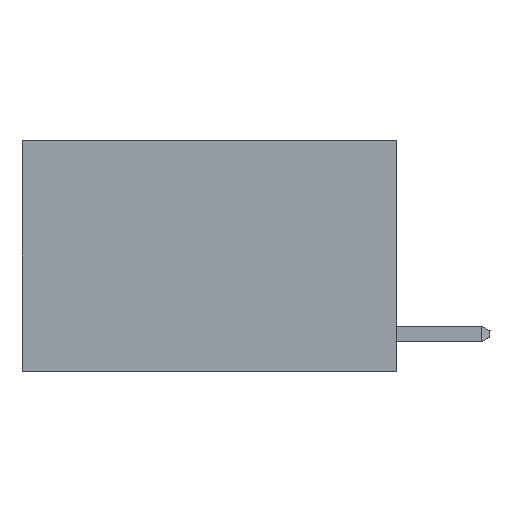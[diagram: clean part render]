
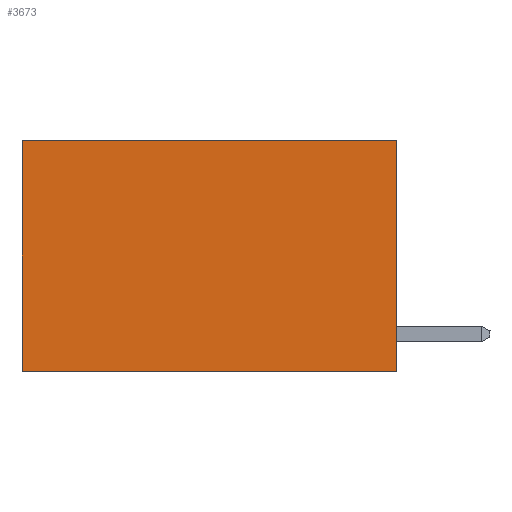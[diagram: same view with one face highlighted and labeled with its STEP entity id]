
A CAD part, left-side view. The second image highlights one B-rep face of the part: STEP entity #3673.
In plain terms, the highlighted planar face has unit normal (-1, 0, 0).
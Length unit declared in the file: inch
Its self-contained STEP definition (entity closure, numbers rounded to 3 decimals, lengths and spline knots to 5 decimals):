
#211 = LINE ( 'NONE', #10325, #7303 ) ;
#1098 = LINE ( 'NONE', #10090, #13282 ) ;
#1186 = PLANE ( 'NONE',  #10611 ) ;
#1551 = ORIENTED_EDGE ( 'NONE', *, *, #12879, .T. ) ;
#2731 = EDGE_LOOP ( 'NONE', ( #1551, #8288, #7806, #10249 ) ) ;
#3109 = VERTEX_POINT ( 'NONE', #12975 ) ;
#3256 = DIRECTION ( 'NONE',  ( 0., 0., -1. ) ) ;
#3499 = CARTESIAN_POINT ( 'NONE',  ( 0.2625, 0., 0. ) ) ;
#3673 = ADVANCED_FACE ( 'NONE', ( #4458 ), #1186, .F. ) ;
#4458 = FACE_OUTER_BOUND ( 'NONE', #2731, .T. ) ;
#4894 = DIRECTION ( 'NONE',  ( 0., 1., 0. ) ) ;
#4955 = VERTEX_POINT ( 'NONE', #10124 ) ;
#5085 = CARTESIAN_POINT ( 'NONE',  ( 0.2625, 0.6, -0.37 ) ) ;
#5705 = DIRECTION ( 'NONE',  ( 0., 0., -1. ) ) ;
#6504 = LINE ( 'NONE', #12105, #10419 ) ;
#6715 = CARTESIAN_POINT ( 'NONE',  ( 0.2625, 0., 0. ) ) ;
#6963 = DIRECTION ( 'NONE',  ( 1., 0., 0. ) ) ;
#7303 = VECTOR ( 'NONE', #4894, 39.37008 ) ;
#7806 = ORIENTED_EDGE ( 'NONE', *, *, #11820, .F. ) ;
#8288 = ORIENTED_EDGE ( 'NONE', *, *, #8401, .F. ) ;
#8401 = EDGE_CURVE ( 'NONE', #4955, #13321, #211, .T. ) ;
#9069 = LINE ( 'NONE', #6715, #12282 ) ;
#9902 = CARTESIAN_POINT ( 'NONE',  ( 0.2625, 0.6, 0. ) ) ;
#10090 = CARTESIAN_POINT ( 'NONE',  ( 0.2625, 0., 0. ) ) ;
#10124 = CARTESIAN_POINT ( 'NONE',  ( 0.2625, 0., -0.37 ) ) ;
#10240 = DIRECTION ( 'NONE',  ( 0., 1., 0. ) ) ;
#10249 = ORIENTED_EDGE ( 'NONE', *, *, #13089, .T. ) ;
#10325 = CARTESIAN_POINT ( 'NONE',  ( 0.2625, 0., -0.37 ) ) ;
#10419 = VECTOR ( 'NONE', #14264, 39.37008 ) ;
#10611 = AXIS2_PLACEMENT_3D ( 'NONE', #3499, #6963, #5705 ) ;
#11820 = EDGE_CURVE ( 'NONE', #3109, #4955, #9069, .T. ) ;
#12105 = CARTESIAN_POINT ( 'NONE',  ( 0.2625, 0.6, 0. ) ) ;
#12282 = VECTOR ( 'NONE', #3256, 39.37008 ) ;
#12879 = EDGE_CURVE ( 'NONE', #13847, #13321, #6504, .T. ) ;
#12975 = CARTESIAN_POINT ( 'NONE',  ( 0.2625, 0., 0. ) ) ;
#13089 = EDGE_CURVE ( 'NONE', #3109, #13847, #1098, .T. ) ;
#13282 = VECTOR ( 'NONE', #10240, 39.37008 ) ;
#13321 = VERTEX_POINT ( 'NONE', #5085 ) ;
#13847 = VERTEX_POINT ( 'NONE', #9902 ) ;
#14264 = DIRECTION ( 'NONE',  ( 0., 0., -1. ) ) ;
